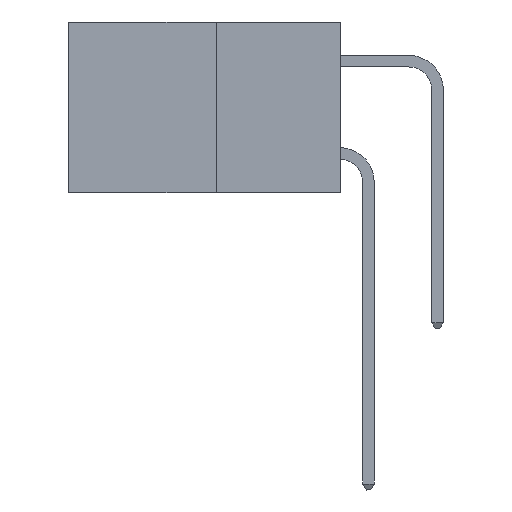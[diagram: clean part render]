
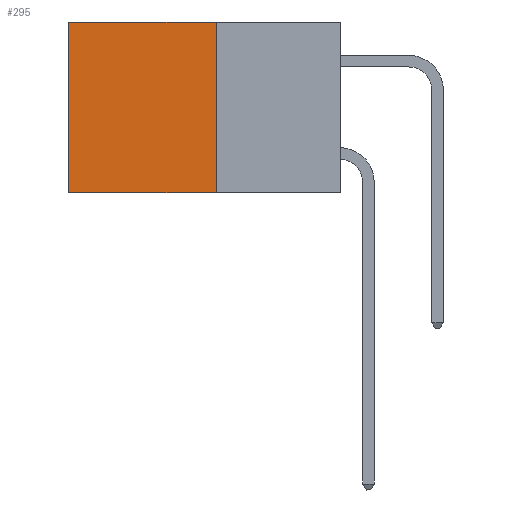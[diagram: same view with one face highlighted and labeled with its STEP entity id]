
A CAD part, left-side view. The second image highlights one B-rep face of the part: STEP entity #295.
In plain terms, the highlighted planar face has unit normal (-1, 0, 0).
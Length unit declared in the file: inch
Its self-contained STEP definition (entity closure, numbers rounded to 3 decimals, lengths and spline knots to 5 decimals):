
#139 = VECTOR ( 'NONE', #11282, 39.37008 ) ;
#295 = ADVANCED_FACE ( 'NONE', ( #800 ), #3362, .F. ) ;
#439 = LINE ( 'NONE', #8419, #139 ) ;
#800 = FACE_OUTER_BOUND ( 'NONE', #3206, .T. ) ;
#850 = DIRECTION ( 'NONE',  ( 0., 0., -1. ) ) ;
#1421 = AXIS2_PLACEMENT_3D ( 'NONE', #3191, #12081, #850 ) ;
#2688 = CARTESIAN_POINT ( 'NONE',  ( 0.277, 0.59, 0. ) ) ;
#3147 = ORIENTED_EDGE ( 'NONE', *, *, #9523, .F. ) ;
#3190 = CARTESIAN_POINT ( 'NONE',  ( 0.277, 0.27, -0.37 ) ) ;
#3191 = CARTESIAN_POINT ( 'NONE',  ( 0.277, 0.27, -0.37 ) ) ;
#3206 = EDGE_LOOP ( 'NONE', ( #8991, #3147, #4625, #5616 ) ) ;
#3362 = PLANE ( 'NONE',  #1421 ) ;
#4625 = ORIENTED_EDGE ( 'NONE', *, *, #6592, .F. ) ;
#4738 = DIRECTION ( 'NONE',  ( 0., 0., -1. ) ) ;
#4946 = VECTOR ( 'NONE', #7879, 39.37008 ) ;
#4976 = VECTOR ( 'NONE', #6501, 39.37008 ) ;
#5261 = LINE ( 'NONE', #12135, #4976 ) ;
#5390 = VERTEX_POINT ( 'NONE', #11405 ) ;
#5616 = ORIENTED_EDGE ( 'NONE', *, *, #11331, .T. ) ;
#6313 = CARTESIAN_POINT ( 'NONE',  ( 0.277, 0.59, -0.37 ) ) ;
#6355 = VECTOR ( 'NONE', #4738, 39.37008 ) ;
#6476 = CARTESIAN_POINT ( 'NONE',  ( 0.277, 0.27, -0.37 ) ) ;
#6501 = DIRECTION ( 'NONE',  ( 0., 1., 0. ) ) ;
#6592 = EDGE_CURVE ( 'NONE', #5390, #7989, #11363, .T. ) ;
#7879 = DIRECTION ( 'NONE',  ( 0., 1., 0. ) ) ;
#7989 = VERTEX_POINT ( 'NONE', #6476 ) ;
#8419 = CARTESIAN_POINT ( 'NONE',  ( 0.277, 0.59, -0.37 ) ) ;
#8456 = VERTEX_POINT ( 'NONE', #6313 ) ;
#8640 = EDGE_CURVE ( 'NONE', #9198, #8456, #439, .T. ) ;
#8991 = ORIENTED_EDGE ( 'NONE', *, *, #8640, .T. ) ;
#9198 = VERTEX_POINT ( 'NONE', #2688 ) ;
#9523 = EDGE_CURVE ( 'NONE', #7989, #8456, #10214, .T. ) ;
#10214 = LINE ( 'NONE', #3190, #4946 ) ;
#10320 = CARTESIAN_POINT ( 'NONE',  ( 0.277, 0.27, -0.37 ) ) ;
#11282 = DIRECTION ( 'NONE',  ( 0., 0., -1. ) ) ;
#11331 = EDGE_CURVE ( 'NONE', #5390, #9198, #5261, .T. ) ;
#11363 = LINE ( 'NONE', #10320, #6355 ) ;
#11405 = CARTESIAN_POINT ( 'NONE',  ( 0.277, 0.27, 0. ) ) ;
#12081 = DIRECTION ( 'NONE',  ( 1., 0., 0. ) ) ;
#12135 = CARTESIAN_POINT ( 'NONE',  ( 0.277, 0.27, 0. ) ) ;
